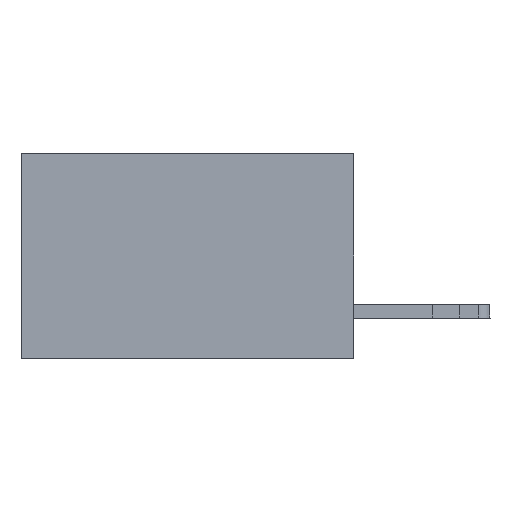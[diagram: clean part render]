
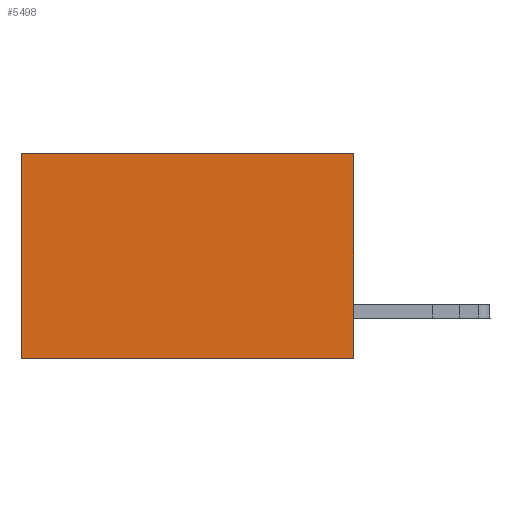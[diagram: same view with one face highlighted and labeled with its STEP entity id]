
A CAD part, left-side view. The second image highlights one B-rep face of the part: STEP entity #5498.
In plain terms, the highlighted planar face has unit normal (-1, 0, 0).
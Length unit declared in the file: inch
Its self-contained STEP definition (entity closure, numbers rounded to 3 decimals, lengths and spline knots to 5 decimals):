
#93 = VECTOR ( 'NONE', #22014, 39.37008 ) ;
#2267 = DIRECTION ( 'NONE',  ( 0., 0., -1. ) ) ;
#2619 = VECTOR ( 'NONE', #26276, 39.37008 ) ;
#2754 = VERTEX_POINT ( 'NONE', #6905 ) ;
#2788 = EDGE_CURVE ( 'NONE', #2754, #16533, #9210, .T. ) ;
#2960 = VECTOR ( 'NONE', #17733, 39.37008 ) ;
#4599 = CARTESIAN_POINT ( 'NONE',  ( 0.2875, 0., -0.37 ) ) ;
#4627 = FACE_OUTER_BOUND ( 'NONE', #25470, .T. ) ;
#5498 = ADVANCED_FACE ( 'NONE', ( #4627 ), #20791, .F. ) ;
#6905 = CARTESIAN_POINT ( 'NONE',  ( 0.2875, 0.6, 0. ) ) ;
#7924 = EDGE_CURVE ( 'NONE', #19563, #16533, #12514, .T. ) ;
#8333 = CARTESIAN_POINT ( 'NONE',  ( 0.2875, 0., 0. ) ) ;
#8757 = ORIENTED_EDGE ( 'NONE', *, *, #7924, .F. ) ;
#8833 = CARTESIAN_POINT ( 'NONE',  ( 0.2875, 0.6, -0.37 ) ) ;
#8904 = LINE ( 'NONE', #11933, #2619 ) ;
#9210 = LINE ( 'NONE', #19721, #2960 ) ;
#9237 = CARTESIAN_POINT ( 'NONE',  ( 0.2875, 0., 0. ) ) ;
#10594 = ORIENTED_EDGE ( 'NONE', *, *, #29450, .F. ) ;
#11933 = CARTESIAN_POINT ( 'NONE',  ( 0.2875, 0., 0. ) ) ;
#12201 = ORIENTED_EDGE ( 'NONE', *, *, #19144, .T. ) ;
#12514 = LINE ( 'NONE', #13222, #93 ) ;
#12670 = DIRECTION ( 'NONE',  ( 0., 1., 0. ) ) ;
#13222 = CARTESIAN_POINT ( 'NONE',  ( 0.2875, 0., -0.37 ) ) ;
#15119 = VECTOR ( 'NONE', #12670, 39.37008 ) ;
#15478 = LINE ( 'NONE', #8333, #15119 ) ;
#16533 = VERTEX_POINT ( 'NONE', #8833 ) ;
#17733 = DIRECTION ( 'NONE',  ( 0., 0., -1. ) ) ;
#19144 = EDGE_CURVE ( 'NONE', #22100, #2754, #15478, .T. ) ;
#19563 = VERTEX_POINT ( 'NONE', #4599 ) ;
#19721 = CARTESIAN_POINT ( 'NONE',  ( 0.2875, 0.6, 0. ) ) ;
#20791 = PLANE ( 'NONE',  #21609 ) ;
#21609 = AXIS2_PLACEMENT_3D ( 'NONE', #9237, #30032, #2267 ) ;
#22014 = DIRECTION ( 'NONE',  ( 0., 1., 0. ) ) ;
#22100 = VERTEX_POINT ( 'NONE', #26137 ) ;
#25470 = EDGE_LOOP ( 'NONE', ( #26896, #8757, #10594, #12201 ) ) ;
#26137 = CARTESIAN_POINT ( 'NONE',  ( 0.2875, 0., 0. ) ) ;
#26276 = DIRECTION ( 'NONE',  ( 0., 0., -1. ) ) ;
#26896 = ORIENTED_EDGE ( 'NONE', *, *, #2788, .T. ) ;
#29450 = EDGE_CURVE ( 'NONE', #22100, #19563, #8904, .T. ) ;
#30032 = DIRECTION ( 'NONE',  ( 1., 0., 0. ) ) ;
